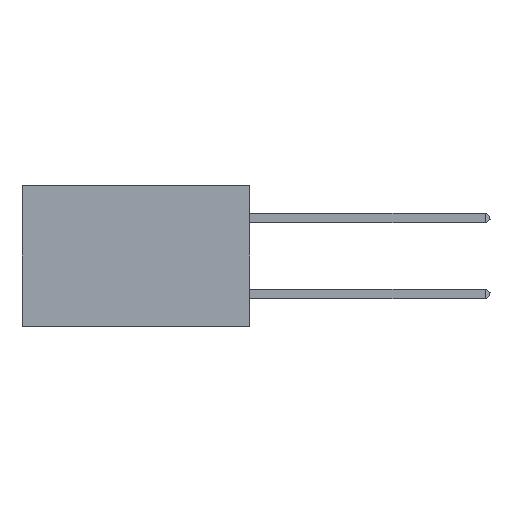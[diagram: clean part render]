
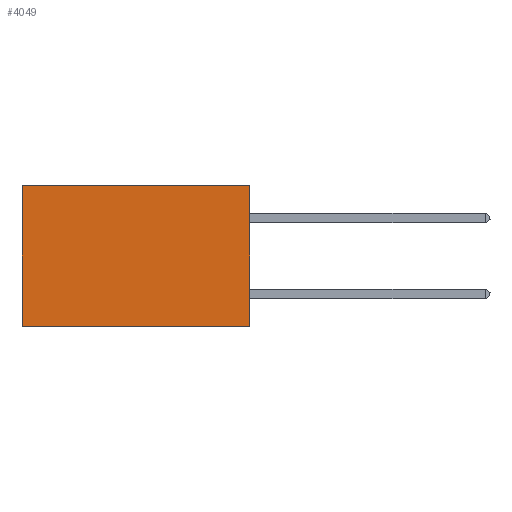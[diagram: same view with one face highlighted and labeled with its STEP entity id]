
A CAD part, left-side view. The second image highlights one B-rep face of the part: STEP entity #4049.
In plain terms, the highlighted planar face has unit normal (-1, 0, 0).
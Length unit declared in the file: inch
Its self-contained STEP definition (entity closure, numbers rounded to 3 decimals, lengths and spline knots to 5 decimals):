
#123 = DIRECTION ( 'NONE',  ( 0., 0., -1. ) ) ;
#1489 = LINE ( 'NONE', #32899, #27369 ) ;
#2348 = DIRECTION ( 'NONE',  ( 0., 1., 0. ) ) ;
#2791 = CARTESIAN_POINT ( 'NONE',  ( 0.2875, 0., 0. ) ) ;
#3709 = AXIS2_PLACEMENT_3D ( 'NONE', #9806, #22876, #4518 ) ;
#4049 = ADVANCED_FACE ( 'NONE', ( #10329 ), #7118, .F. ) ;
#4518 = DIRECTION ( 'NONE',  ( 0., 0., -1. ) ) ;
#4532 = CARTESIAN_POINT ( 'NONE',  ( 0.2875, 0.6, 0. ) ) ;
#4722 = EDGE_CURVE ( 'NONE', #20277, #17026, #1489, .T. ) ;
#4926 = ORIENTED_EDGE ( 'NONE', *, *, #4722, .F. ) ;
#6566 = LINE ( 'NONE', #2791, #28241 ) ;
#7118 = PLANE ( 'NONE',  #3709 ) ;
#9253 = EDGE_CURVE ( 'NONE', #10714, #20277, #23891, .T. ) ;
#9806 = CARTESIAN_POINT ( 'NONE',  ( 0.2875, 0., 0. ) ) ;
#10329 = FACE_OUTER_BOUND ( 'NONE', #25232, .T. ) ;
#10328 = CARTESIAN_POINT ( 'NONE',  ( 0.2875, 0., 0. ) ) ;
#10714 = VERTEX_POINT ( 'NONE', #14846 ) ;
#11017 = CARTESIAN_POINT ( 'NONE',  ( 0.2875, 0., -0.37 ) ) ;
#11293 = VECTOR ( 'NONE', #123, 39.37008 ) ;
#12015 = VERTEX_POINT ( 'NONE', #4532 ) ;
#14425 = EDGE_CURVE ( 'NONE', #12015, #17026, #25505, .T. ) ;
#14846 = CARTESIAN_POINT ( 'NONE',  ( 0.2875, 0., 0. ) ) ;
#15245 = ORIENTED_EDGE ( 'NONE', *, *, #14425, .T. ) ;
#16218 = CARTESIAN_POINT ( 'NONE',  ( 0.2875, 0.6, 0. ) ) ;
#17026 = VERTEX_POINT ( 'NONE', #23484 ) ;
#17243 = VECTOR ( 'NONE', #26336, 39.37008 ) ;
#17363 = ORIENTED_EDGE ( 'NONE', *, *, #20667, .T. ) ;
#18801 = ORIENTED_EDGE ( 'NONE', *, *, #9253, .F. ) ;
#20277 = VERTEX_POINT ( 'NONE', #11017 ) ;
#20667 = EDGE_CURVE ( 'NONE', #10714, #12015, #6566, .T. ) ;
#22876 = DIRECTION ( 'NONE',  ( 1., 0., 0. ) ) ;
#23484 = CARTESIAN_POINT ( 'NONE',  ( 0.2875, 0.6, -0.37 ) ) ;
#23891 = LINE ( 'NONE', #10328, #17243 ) ;
#25047 = DIRECTION ( 'NONE',  ( 0., 1., 0. ) ) ;
#25232 = EDGE_LOOP ( 'NONE', ( #15245, #4926, #18801, #17363 ) ) ;
#25505 = LINE ( 'NONE', #16218, #11293 ) ;
#26336 = DIRECTION ( 'NONE',  ( 0., 0., -1. ) ) ;
#27369 = VECTOR ( 'NONE', #25047, 39.37008 ) ;
#28241 = VECTOR ( 'NONE', #2348, 39.37008 ) ;
#32899 = CARTESIAN_POINT ( 'NONE',  ( 0.2875, 0., -0.37 ) ) ;
